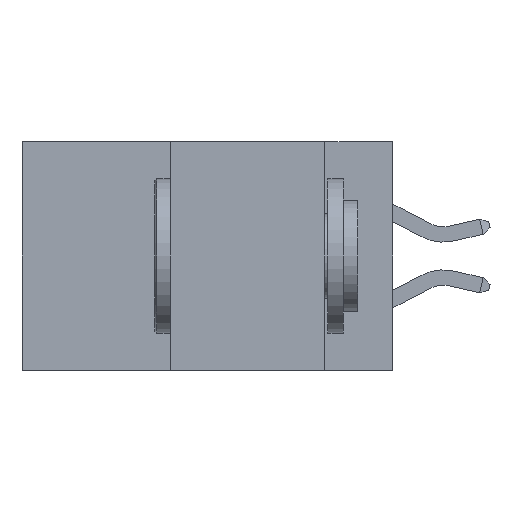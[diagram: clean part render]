
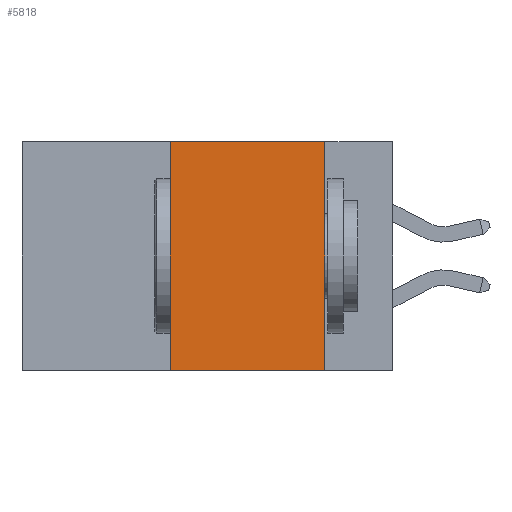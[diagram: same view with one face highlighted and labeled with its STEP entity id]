
A CAD part, left-side view. The second image highlights one B-rep face of the part: STEP entity #5818.
In plain terms, the highlighted planar face has unit normal (-1, 0, 0).
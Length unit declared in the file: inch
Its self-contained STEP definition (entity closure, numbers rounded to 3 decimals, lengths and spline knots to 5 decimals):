
#60 = DIRECTION ( 'NONE',  ( 0., 0., -1. ) ) ;
#334 = CARTESIAN_POINT ( 'NONE',  ( 0., 0.36, 0. ) ) ;
#340 = AXIS2_PLACEMENT_3D ( 'NONE', #11871, #6710, #60 ) ;
#857 = DIRECTION ( 'NONE',  ( 0., -1., 0. ) ) ;
#873 = CARTESIAN_POINT ( 'NONE',  ( 0., 0.11, -0.37 ) ) ;
#1391 = LINE ( 'NONE', #12007, #21493 ) ;
#2417 = LINE ( 'NONE', #12319, #3977 ) ;
#3160 = DIRECTION ( 'NONE',  ( 0., -1., 0. ) ) ;
#3656 = DIRECTION ( 'NONE',  ( 0., 0., -1. ) ) ;
#3854 = EDGE_CURVE ( 'NONE', #17056, #11036, #1391, .T. ) ;
#3977 = VECTOR ( 'NONE', #857, 39.37008 ) ;
#5818 = ADVANCED_FACE ( 'NONE', ( #10469 ), #13154, .F. ) ;
#5851 = CARTESIAN_POINT ( 'NONE',  ( 0., 0.11, 0. ) ) ;
#6710 = DIRECTION ( 'NONE',  ( 1., 0., 0. ) ) ;
#7404 = ORIENTED_EDGE ( 'NONE', *, *, #21576, .F. ) ;
#7674 = CARTESIAN_POINT ( 'NONE',  ( 0., 0.6, -0.37 ) ) ;
#8986 = CARTESIAN_POINT ( 'NONE',  ( 0., 0.11, 0. ) ) ;
#9107 = VERTEX_POINT ( 'NONE', #873 ) ;
#10352 = ORIENTED_EDGE ( 'NONE', *, *, #3854, .F. ) ;
#10469 = FACE_OUTER_BOUND ( 'NONE', #17208, .T. ) ;
#10836 = LINE ( 'NONE', #7674, #19425 ) ;
#11036 = VERTEX_POINT ( 'NONE', #334 ) ;
#11871 = CARTESIAN_POINT ( 'NONE',  ( 0., 0.6, 0. ) ) ;
#12007 = CARTESIAN_POINT ( 'NONE',  ( 0., 0.36, 0. ) ) ;
#12319 = CARTESIAN_POINT ( 'NONE',  ( 0., 0.6, 0. ) ) ;
#12599 = VERTEX_POINT ( 'NONE', #5851 ) ;
#13154 = PLANE ( 'NONE',  #340 ) ;
#13705 = VECTOR ( 'NONE', #3656, 39.37008 ) ;
#13867 = DIRECTION ( 'NONE',  ( 0., 0., 1. ) ) ;
#15627 = ORIENTED_EDGE ( 'NONE', *, *, #19819, .T. ) ;
#16495 = ORIENTED_EDGE ( 'NONE', *, *, #16579, .F. ) ;
#16579 = EDGE_CURVE ( 'NONE', #12599, #9107, #17865, .T. ) ;
#17056 = VERTEX_POINT ( 'NONE', #20146 ) ;
#17208 = EDGE_LOOP ( 'NONE', ( #16495, #7404, #10352, #15627 ) ) ;
#17865 = LINE ( 'NONE', #8986, #13705 ) ;
#19425 = VECTOR ( 'NONE', #3160, 39.37008 ) ;
#19819 = EDGE_CURVE ( 'NONE', #17056, #9107, #10836, .T. ) ;
#20146 = CARTESIAN_POINT ( 'NONE',  ( 0., 0.36, -0.37 ) ) ;
#21493 = VECTOR ( 'NONE', #13867, 39.37008 ) ;
#21576 = EDGE_CURVE ( 'NONE', #11036, #12599, #2417, .T. ) ;
